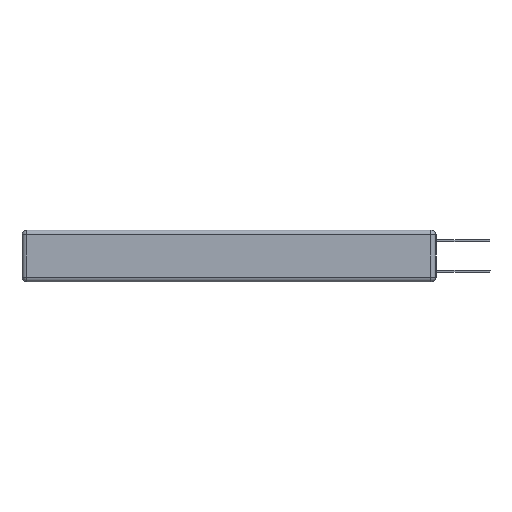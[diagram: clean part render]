
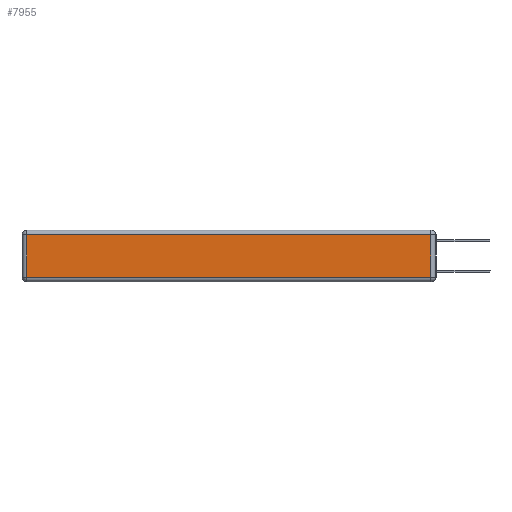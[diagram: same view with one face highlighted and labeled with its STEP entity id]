
A CAD part, left-side view. The second image highlights one B-rep face of the part: STEP entity #7955.
In plain terms, the highlighted planar face has unit normal (-1, 0, 0).
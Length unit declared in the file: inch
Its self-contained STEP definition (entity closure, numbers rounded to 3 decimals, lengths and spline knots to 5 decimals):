
#288 = CARTESIAN_POINT ( 'NONE',  ( 0., 0.03, -0.343 ) ) ;
#987 = CARTESIAN_POINT ( 'NONE',  ( 0., 2.75, -0.03 ) ) ;
#1458 = CARTESIAN_POINT ( 'NONE',  ( 0., 0.03, -0.03 ) ) ;
#1999 = DIRECTION ( 'NONE',  ( 0., 1., 0. ) ) ;
#3293 = ORIENTED_EDGE ( 'NONE', *, *, #10838, .T. ) ;
#3351 = VERTEX_POINT ( 'NONE', #1458 ) ;
#3871 = EDGE_CURVE ( 'NONE', #9859, #11436, #12744, .T. ) ;
#4142 = AXIS2_PLACEMENT_3D ( 'NONE', #11085, #7928, #7971 ) ;
#4482 = EDGE_LOOP ( 'NONE', ( #9382, #4530, #9727, #3293 ) ) ;
#4530 = ORIENTED_EDGE ( 'NONE', *, *, #6538, .T. ) ;
#6020 = CARTESIAN_POINT ( 'NONE',  ( 0., 2.72, -0.313 ) ) ;
#6431 = VECTOR ( 'NONE', #12564, 39.37008 ) ;
#6538 = EDGE_CURVE ( 'NONE', #11436, #3351, #9098, .T. ) ;
#6673 = VECTOR ( 'NONE', #11539, 39.37008 ) ;
#7477 = VERTEX_POINT ( 'NONE', #9013 ) ;
#7928 = DIRECTION ( 'NONE',  ( -1., 0., 0. ) ) ;
#7955 = ADVANCED_FACE ( 'NONE', ( #12288 ), #12047, .T. ) ;
#7971 = DIRECTION ( 'NONE',  ( 0., 0., 1. ) ) ;
#8266 = CARTESIAN_POINT ( 'NONE',  ( 0., 0.03, -0.313 ) ) ;
#8547 = VECTOR ( 'NONE', #9815, 39.37008 ) ;
#8814 = LINE ( 'NONE', #987, #12854 ) ;
#9013 = CARTESIAN_POINT ( 'NONE',  ( 0., 2.72, -0.03 ) ) ;
#9098 = LINE ( 'NONE', #288, #6431 ) ;
#9382 = ORIENTED_EDGE ( 'NONE', *, *, #3871, .T. ) ;
#9727 = ORIENTED_EDGE ( 'NONE', *, *, #13211, .T. ) ;
#9815 = DIRECTION ( 'NONE',  ( 0., 0., -1. ) ) ;
#9840 = LINE ( 'NONE', #11796, #8547 ) ;
#9859 = VERTEX_POINT ( 'NONE', #6020 ) ;
#10567 = CARTESIAN_POINT ( 'NONE',  ( 0., 0., -0.313 ) ) ;
#10838 = EDGE_CURVE ( 'NONE', #7477, #9859, #9840, .T. ) ;
#11085 = CARTESIAN_POINT ( 'NONE',  ( 0., 0., -0.343 ) ) ;
#11436 = VERTEX_POINT ( 'NONE', #8266 ) ;
#11539 = DIRECTION ( 'NONE',  ( 0., -1., 0. ) ) ;
#11796 = CARTESIAN_POINT ( 'NONE',  ( 0., 2.72, -0.343 ) ) ;
#12047 = PLANE ( 'NONE',  #4142 ) ;
#12288 = FACE_OUTER_BOUND ( 'NONE', #4482, .T. ) ;
#12564 = DIRECTION ( 'NONE',  ( 0., 0., 1. ) ) ;
#12744 = LINE ( 'NONE', #10567, #6673 ) ;
#12854 = VECTOR ( 'NONE', #1999, 39.37008 ) ;
#13211 = EDGE_CURVE ( 'NONE', #3351, #7477, #8814, .T. ) ;
